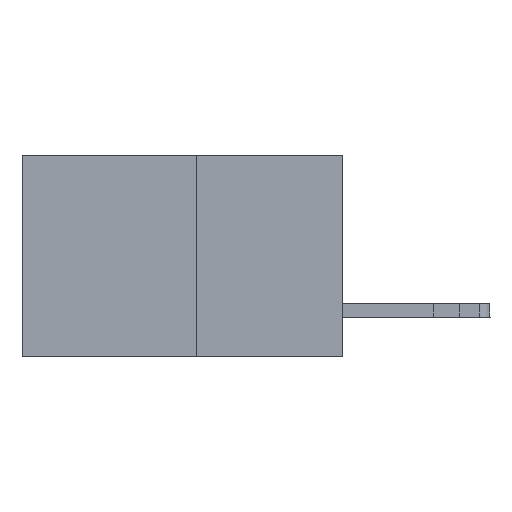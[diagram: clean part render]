
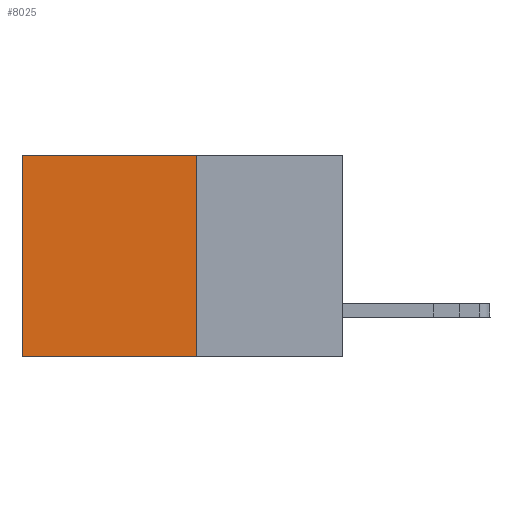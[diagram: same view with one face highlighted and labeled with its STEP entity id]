
A CAD part, left-side view. The second image highlights one B-rep face of the part: STEP entity #8025.
In plain terms, the highlighted planar face has unit normal (-1, 0, 0).
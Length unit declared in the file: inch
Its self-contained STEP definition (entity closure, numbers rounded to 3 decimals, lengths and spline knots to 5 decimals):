
#197 = DIRECTION ( 'NONE',  ( 1., 0., 0. ) ) ;
#283 = EDGE_CURVE ( 'NONE', #9737, #5128, #5285, .T. ) ;
#1767 = DIRECTION ( 'NONE',  ( 0., 1., 0. ) ) ;
#3537 = LINE ( 'NONE', #7459, #10558 ) ;
#5128 = VERTEX_POINT ( 'NONE', #15598 ) ;
#5285 = LINE ( 'NONE', #12815, #8999 ) ;
#5666 = AXIS2_PLACEMENT_3D ( 'NONE', #17149, #197, #10185 ) ;
#5676 = CARTESIAN_POINT ( 'NONE',  ( 0.277, 0.59, 0. ) ) ;
#5866 = CARTESIAN_POINT ( 'NONE',  ( 0.277, 0.27, 0. ) ) ;
#6662 = VECTOR ( 'NONE', #1767, 39.37008 ) ;
#7258 = DIRECTION ( 'NONE',  ( 0., 1., 0. ) ) ;
#7368 = PLANE ( 'NONE',  #5666 ) ;
#7429 = ORIENTED_EDGE ( 'NONE', *, *, #283, .T. ) ;
#7459 = CARTESIAN_POINT ( 'NONE',  ( 0.277, 0.27, -0.37 ) ) ;
#8025 = ADVANCED_FACE ( 'NONE', ( #15146 ), #7368, .F. ) ;
#8999 = VECTOR ( 'NONE', #14629, 39.37008 ) ;
#9370 = ORIENTED_EDGE ( 'NONE', *, *, #10616, .F. ) ;
#9737 = VERTEX_POINT ( 'NONE', #5676 ) ;
#9818 = ORIENTED_EDGE ( 'NONE', *, *, #12549, .F. ) ;
#9947 = ORIENTED_EDGE ( 'NONE', *, *, #13942, .T. ) ;
#10185 = DIRECTION ( 'NONE',  ( 0., 0., -1. ) ) ;
#10276 = DIRECTION ( 'NONE',  ( 0., 0., -1. ) ) ;
#10558 = VECTOR ( 'NONE', #10276, 39.37008 ) ;
#10616 = EDGE_CURVE ( 'NONE', #17397, #5128, #14189, .T. ) ;
#11370 = VECTOR ( 'NONE', #7258, 39.37008 ) ;
#11575 = CARTESIAN_POINT ( 'NONE',  ( 0.277, 0.27, -0.37 ) ) ;
#11828 = LINE ( 'NONE', #5866, #11370 ) ;
#12549 = EDGE_CURVE ( 'NONE', #15139, #17397, #3537, .T. ) ;
#12815 = CARTESIAN_POINT ( 'NONE',  ( 0.277, 0.59, -0.37 ) ) ;
#13362 = EDGE_LOOP ( 'NONE', ( #7429, #9370, #9818, #9947 ) ) ;
#13942 = EDGE_CURVE ( 'NONE', #15139, #9737, #11828, .T. ) ;
#14189 = LINE ( 'NONE', #11575, #6662 ) ;
#14629 = DIRECTION ( 'NONE',  ( 0., 0., -1. ) ) ;
#15139 = VERTEX_POINT ( 'NONE', #15653 ) ;
#15146 = FACE_OUTER_BOUND ( 'NONE', #13362, .T. ) ;
#15266 = CARTESIAN_POINT ( 'NONE',  ( 0.277, 0.27, -0.37 ) ) ;
#15598 = CARTESIAN_POINT ( 'NONE',  ( 0.277, 0.59, -0.37 ) ) ;
#15653 = CARTESIAN_POINT ( 'NONE',  ( 0.277, 0.27, 0. ) ) ;
#17149 = CARTESIAN_POINT ( 'NONE',  ( 0.277, 0.27, -0.37 ) ) ;
#17397 = VERTEX_POINT ( 'NONE', #15266 ) ;
